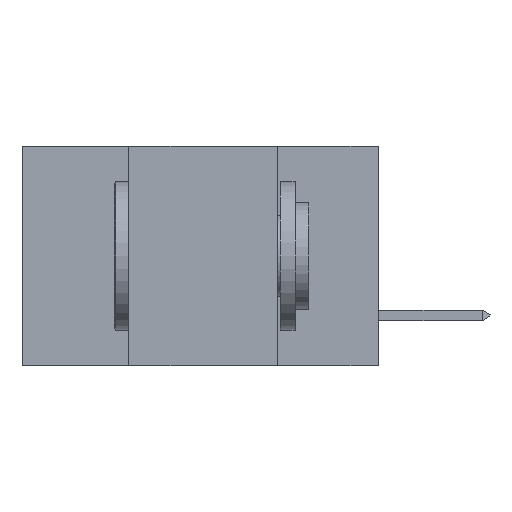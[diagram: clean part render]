
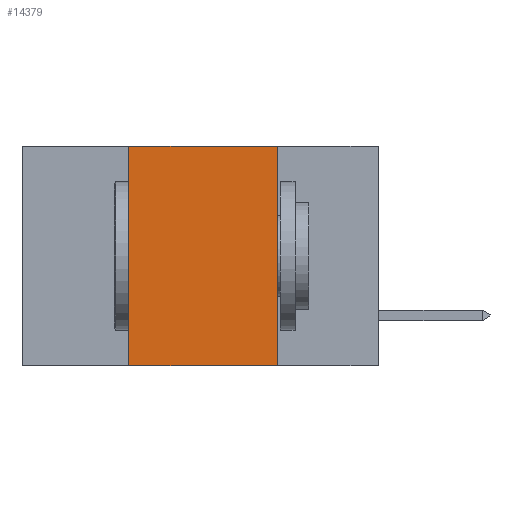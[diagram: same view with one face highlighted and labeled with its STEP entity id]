
A CAD part, left-side view. The second image highlights one B-rep face of the part: STEP entity #14379.
In plain terms, the highlighted planar face has unit normal (-1, 0, 0).
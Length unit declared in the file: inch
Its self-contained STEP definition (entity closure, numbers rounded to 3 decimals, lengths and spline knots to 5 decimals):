
#379 = CARTESIAN_POINT ( 'NONE',  ( 0., 0.42, -0.37 ) ) ;
#841 = FACE_OUTER_BOUND ( 'NONE', #8217, .T. ) ;
#1481 = CARTESIAN_POINT ( 'NONE',  ( 0., 0.17, -0.37 ) ) ;
#1502 = VERTEX_POINT ( 'NONE', #379 ) ;
#1801 = ORIENTED_EDGE ( 'NONE', *, *, #11944, .F. ) ;
#2633 = EDGE_CURVE ( 'NONE', #1502, #9750, #10294, .T. ) ;
#3533 = CARTESIAN_POINT ( 'NONE',  ( 0., 0.6, 0. ) ) ;
#3798 = VERTEX_POINT ( 'NONE', #8862 ) ;
#5290 = CARTESIAN_POINT ( 'NONE',  ( 0., 0.17, 0. ) ) ;
#5357 = VECTOR ( 'NONE', #9521, 39.37008 ) ;
#5781 = ORIENTED_EDGE ( 'NONE', *, *, #14684, .F. ) ;
#6072 = ORIENTED_EDGE ( 'NONE', *, *, #11384, .F. ) ;
#6487 = PLANE ( 'NONE',  #15961 ) ;
#6827 = ORIENTED_EDGE ( 'NONE', *, *, #2633, .T. ) ;
#7402 = VECTOR ( 'NONE', #9633, 39.37008 ) ;
#7895 = LINE ( 'NONE', #3533, #17099 ) ;
#8217 = EDGE_LOOP ( 'NONE', ( #1801, #6072, #5781, #6827 ) ) ;
#8256 = VECTOR ( 'NONE', #9178, 39.37008 ) ;
#8761 = CARTESIAN_POINT ( 'NONE',  ( 0., 0.17, 0. ) ) ;
#8862 = CARTESIAN_POINT ( 'NONE',  ( 0., 0.42, 0. ) ) ;
#9178 = DIRECTION ( 'NONE',  ( 0., -1., 0. ) ) ;
#9397 = CARTESIAN_POINT ( 'NONE',  ( 0., 0.6, 0. ) ) ;
#9521 = DIRECTION ( 'NONE',  ( 0., 0., -1. ) ) ;
#9633 = DIRECTION ( 'NONE',  ( 0., 0., 1. ) ) ;
#9750 = VERTEX_POINT ( 'NONE', #1481 ) ;
#10294 = LINE ( 'NONE', #15722, #8256 ) ;
#11384 = EDGE_CURVE ( 'NONE', #3798, #12007, #7895, .T. ) ;
#11944 = EDGE_CURVE ( 'NONE', #12007, #9750, #12780, .T. ) ;
#12007 = VERTEX_POINT ( 'NONE', #8761 ) ;
#12780 = LINE ( 'NONE', #5290, #5357 ) ;
#13716 = DIRECTION ( 'NONE',  ( 1., 0., 0. ) ) ;
#13782 = CARTESIAN_POINT ( 'NONE',  ( 0., 0.42, 0. ) ) ;
#14379 = ADVANCED_FACE ( 'NONE', ( #841 ), #6487, .F. ) ;
#14684 = EDGE_CURVE ( 'NONE', #1502, #3798, #17516, .T. ) ;
#15722 = CARTESIAN_POINT ( 'NONE',  ( 0., 0.6, -0.37 ) ) ;
#15961 = AXIS2_PLACEMENT_3D ( 'NONE', #9397, #13716, #18060 ) ;
#17099 = VECTOR ( 'NONE', #17803, 39.37008 ) ;
#17516 = LINE ( 'NONE', #13782, #7402 ) ;
#17803 = DIRECTION ( 'NONE',  ( 0., -1., 0. ) ) ;
#18060 = DIRECTION ( 'NONE',  ( 0., 0., -1. ) ) ;
